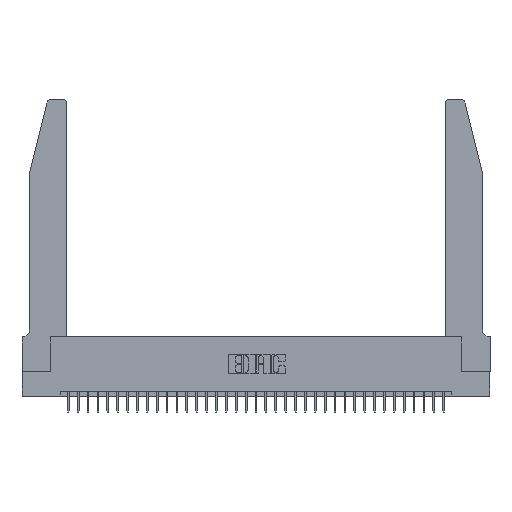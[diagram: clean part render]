
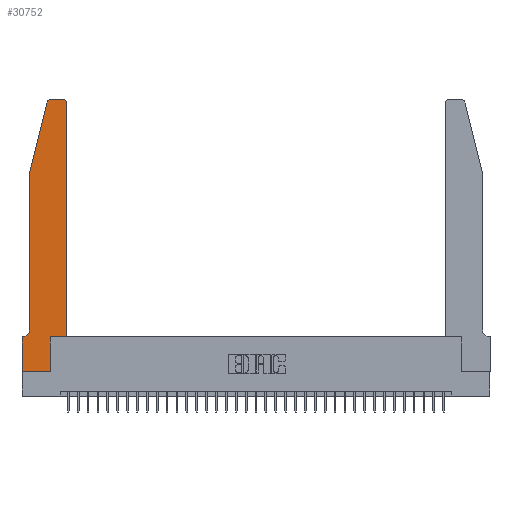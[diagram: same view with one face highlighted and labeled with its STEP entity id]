
A CAD part, top view. The second image highlights one B-rep face of the part: STEP entity #30752.
In plain terms, the highlighted planar face has unit normal (0, 0, 1).
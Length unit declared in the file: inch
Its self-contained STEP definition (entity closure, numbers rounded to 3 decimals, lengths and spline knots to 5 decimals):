
#19 = VERTEX_POINT ( 'NONE', #4647 ) ;
#34 = CARTESIAN_POINT ( 'NONE',  ( 0.4205, 2.75, 0.37 ) ) ;
#842 = LINE ( 'NONE', #7567, #33002 ) ;
#1117 = EDGE_CURVE ( 'NONE', #4156, #19, #4498, .T. ) ;
#1240 = VERTEX_POINT ( 'NONE', #16334 ) ;
#1592 = CARTESIAN_POINT ( 'NONE',  ( 0.0755, 2., 0.37 ) ) ;
#2178 = CARTESIAN_POINT ( 'NONE',  ( 0., 0., 0.37 ) ) ;
#2270 = CARTESIAN_POINT ( 'NONE',  ( 0., 0., 0.37 ) ) ;
#2315 = ORIENTED_EDGE ( 'NONE', *, *, #11232, .T. ) ;
#2778 = AXIS2_PLACEMENT_3D ( 'NONE', #22079, #33148, #30562 ) ;
#3242 = EDGE_CURVE ( 'NONE', #3305, #18159, #8334, .T. ) ;
#3296 = VECTOR ( 'NONE', #25393, 39.37008 ) ;
#3305 = VERTEX_POINT ( 'NONE', #27354 ) ;
#3599 = CARTESIAN_POINT ( 'NONE',  ( 0.2605, 2.75, 0.37 ) ) ;
#4156 = VERTEX_POINT ( 'NONE', #31118 ) ;
#4162 = VECTOR ( 'NONE', #29363, 39.37008 ) ;
#4498 = LINE ( 'NONE', #2178, #11058 ) ;
#4647 = CARTESIAN_POINT ( 'NONE',  ( 0., 0., 0.37 ) ) ;
#4722 = VERTEX_POINT ( 'NONE', #34 ) ;
#4886 = DIRECTION ( 'NONE',  ( 1., 0., 0. ) ) ;
#4969 = DIRECTION ( 'NONE',  ( -0.239, -0.971, 0. ) ) ;
#5169 = DIRECTION ( 'NONE',  ( 0., 0., 1. ) ) ;
#5546 = PLANE ( 'NONE',  #2778 ) ;
#6254 = CARTESIAN_POINT ( 'NONE',  ( 0.0055, 0.35, 0.37 ) ) ;
#6444 = LINE ( 'NONE', #2270, #23310 ) ;
#7567 = CARTESIAN_POINT ( 'NONE',  ( 0.4505, 0.35, 0.37 ) ) ;
#8334 = LINE ( 'NONE', #27119, #20296 ) ;
#8434 = EDGE_CURVE ( 'NONE', #19, #3305, #6444, .T. ) ;
#8499 = FACE_OUTER_BOUND ( 'NONE', #13152, .T. ) ;
#8558 = LINE ( 'NONE', #3599, #3296 ) ;
#8880 = ORIENTED_EDGE ( 'NONE', *, *, #29635, .T. ) ;
#9177 = CIRCLE ( 'NONE', #19797, 0.07 ) ;
#9785 = CARTESIAN_POINT ( 'NONE',  ( 0.4505, 0.35, 0.37 ) ) ;
#10109 = LINE ( 'NONE', #26455, #30428 ) ;
#11058 = VECTOR ( 'NONE', #35491, 39.37008 ) ;
#11232 = EDGE_CURVE ( 'NONE', #24759, #30390, #15824, .T. ) ;
#11706 = ORIENTED_EDGE ( 'NONE', *, *, #8434, .T. ) ;
#11843 = CARTESIAN_POINT ( 'NONE',  ( 0.25487, 2.72718, 0.37 ) ) ;
#12174 = VECTOR ( 'NONE', #24185, 39.37008 ) ;
#13152 = EDGE_LOOP ( 'NONE', ( #8880, #21151, #14569, #2315, #20516, #29161, #13819, #11706, #18682, #16914, #23757, #18998 ) ) ;
#13819 = ORIENTED_EDGE ( 'NONE', *, *, #1117, .T. ) ;
#14298 = CARTESIAN_POINT ( 'NONE',  ( 0.4505, 2.72, 0.37 ) ) ;
#14569 = ORIENTED_EDGE ( 'NONE', *, *, #25903, .T. ) ;
#15317 = EDGE_CURVE ( 'NONE', #30013, #32172, #33778, .T. ) ;
#15519 = DIRECTION ( 'NONE',  ( 0., 0., -1. ) ) ;
#15640 = CARTESIAN_POINT ( 'NONE',  ( 0.0055, 0.42, 0.37 ) ) ;
#15747 = DIRECTION ( 'NONE',  ( -1., 0., 0. ) ) ;
#15824 = LINE ( 'NONE', #21734, #32297 ) ;
#15971 = EDGE_CURVE ( 'NONE', #32327, #4722, #33724, .T. ) ;
#16105 = CARTESIAN_POINT ( 'NONE',  ( 0.284, 2.75, 0.37 ) ) ;
#16163 = CARTESIAN_POINT ( 'NONE',  ( 0.284, 2.72, 0.37 ) ) ;
#16334 = CARTESIAN_POINT ( 'NONE',  ( 0.4505, 0.35, 0.37 ) ) ;
#16914 = ORIENTED_EDGE ( 'NONE', *, *, #26487, .T. ) ;
#17120 = LINE ( 'NONE', #9785, #4162 ) ;
#17175 = EDGE_CURVE ( 'NONE', #1240, #32327, #17120, .T. ) ;
#18159 = VERTEX_POINT ( 'NONE', #20677 ) ;
#18682 = ORIENTED_EDGE ( 'NONE', *, *, #3242, .T. ) ;
#18998 = ORIENTED_EDGE ( 'NONE', *, *, #15971, .T. ) ;
#19109 = DIRECTION ( 'NONE',  ( 0., 1., 0. ) ) ;
#19797 = AXIS2_PLACEMENT_3D ( 'NONE', #15640, #15519, #15747 ) ;
#19838 = CARTESIAN_POINT ( 'NONE',  ( 0.4205, 2.72, 0.37 ) ) ;
#20296 = VECTOR ( 'NONE', #19109, 39.37008 ) ;
#20516 = ORIENTED_EDGE ( 'NONE', *, *, #26478, .T. ) ;
#20677 = CARTESIAN_POINT ( 'NONE',  ( 0.2865, 0.35, 0.37 ) ) ;
#21035 = AXIS2_PLACEMENT_3D ( 'NONE', #16163, #5169, #27293 ) ;
#21151 = ORIENTED_EDGE ( 'NONE', *, *, #15317, .T. ) ;
#21358 = DIRECTION ( 'NONE',  ( 0., -1., 0. ) ) ;
#21734 = CARTESIAN_POINT ( 'NONE',  ( 0.0755, 2., 0.37 ) ) ;
#22079 = CARTESIAN_POINT ( 'NONE',  ( 0., 0.35, 0.37 ) ) ;
#23310 = VECTOR ( 'NONE', #30582, 39.37008 ) ;
#23669 = CARTESIAN_POINT ( 'NONE',  ( 0.0755, 0.35, 0.37 ) ) ;
#23757 = ORIENTED_EDGE ( 'NONE', *, *, #17175, .T. ) ;
#24185 = DIRECTION ( 'NONE',  ( -1., 0., 0. ) ) ;
#24759 = VERTEX_POINT ( 'NONE', #1592 ) ;
#25105 = DIRECTION ( 'NONE',  ( 0., 0., 1. ) ) ;
#25393 = DIRECTION ( 'NONE',  ( -1., 0., 0. ) ) ;
#25680 = AXIS2_PLACEMENT_3D ( 'NONE', #19838, #25105, #27897 ) ;
#25903 = EDGE_CURVE ( 'NONE', #32172, #24759, #10109, .T. ) ;
#26455 = CARTESIAN_POINT ( 'NONE',  ( 0.0755, 2., 0.37 ) ) ;
#26478 = EDGE_CURVE ( 'NONE', #30390, #30281, #9177, .T. ) ;
#26487 = EDGE_CURVE ( 'NONE', #18159, #1240, #842, .T. ) ;
#26873 = LINE ( 'NONE', #23669, #12174 ) ;
#26940 = EDGE_CURVE ( 'NONE', #30281, #4156, #26873, .T. ) ;
#27119 = CARTESIAN_POINT ( 'NONE',  ( 0.2865, 0.35, 0.37 ) ) ;
#27293 = DIRECTION ( 'NONE',  ( 1., 0., 0. ) ) ;
#27354 = CARTESIAN_POINT ( 'NONE',  ( 0.2865, 0., 0.37 ) ) ;
#27897 = DIRECTION ( 'NONE',  ( 1., 0., 0. ) ) ;
#29161 = ORIENTED_EDGE ( 'NONE', *, *, #26940, .T. ) ;
#29363 = DIRECTION ( 'NONE',  ( 0., 1., 0. ) ) ;
#29635 = EDGE_CURVE ( 'NONE', #4722, #30013, #8558, .T. ) ;
#30013 = VERTEX_POINT ( 'NONE', #16105 ) ;
#30281 = VERTEX_POINT ( 'NONE', #6254 ) ;
#30390 = VERTEX_POINT ( 'NONE', #31045 ) ;
#30428 = VECTOR ( 'NONE', #4969, 39.37008 ) ;
#30562 = DIRECTION ( 'NONE',  ( 1., 0., 0. ) ) ;
#30582 = DIRECTION ( 'NONE',  ( 1., 0., 0. ) ) ;
#30752 = ADVANCED_FACE ( 'NONE', ( #8499 ), #5546, .T. ) ;
#31045 = CARTESIAN_POINT ( 'NONE',  ( 0.0755, 0.42, 0.37 ) ) ;
#31118 = CARTESIAN_POINT ( 'NONE',  ( 0., 0.35, 0.37 ) ) ;
#32172 = VERTEX_POINT ( 'NONE', #11843 ) ;
#32297 = VECTOR ( 'NONE', #21358, 39.37008 ) ;
#32327 = VERTEX_POINT ( 'NONE', #14298 ) ;
#33002 = VECTOR ( 'NONE', #4886, 39.37008 ) ;
#33148 = DIRECTION ( 'NONE',  ( 0., 0., 1. ) ) ;
#33724 = CIRCLE ( 'NONE', #25680, 0.03 ) ;
#33778 = CIRCLE ( 'NONE', #21035, 0.03 ) ;
#35491 = DIRECTION ( 'NONE',  ( 0., -1., 0. ) ) ;
